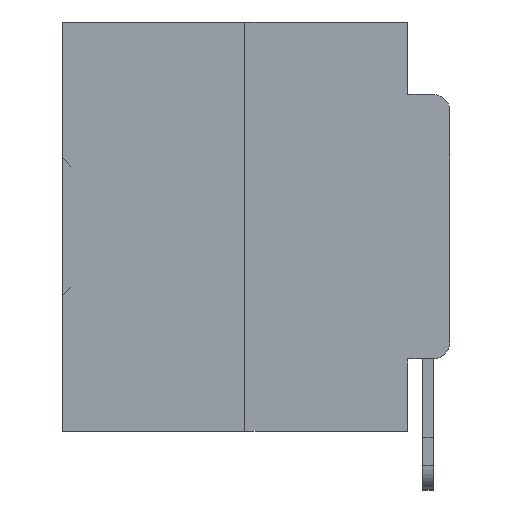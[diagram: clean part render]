
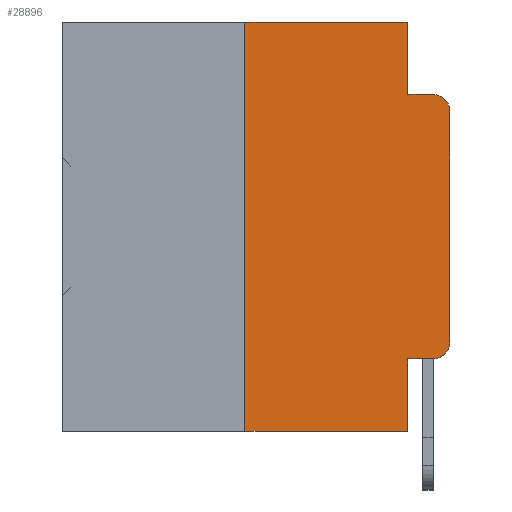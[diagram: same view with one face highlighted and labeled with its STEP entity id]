
A CAD part, left-side view. The second image highlights one B-rep face of the part: STEP entity #28896.
In plain terms, the highlighted planar face has unit normal (-1, 0, 0).
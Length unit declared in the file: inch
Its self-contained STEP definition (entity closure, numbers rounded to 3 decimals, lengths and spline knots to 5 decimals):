
#192 = DIRECTION ( 'NONE',  ( -1., 0., 0. ) ) ;
#407 = VERTEX_POINT ( 'NONE', #36374 ) ;
#588 = VERTEX_POINT ( 'NONE', #10167 ) ;
#618 = AXIS2_PLACEMENT_3D ( 'NONE', #33486, #6969, #27730 ) ;
#1060 = FACE_OUTER_BOUND ( 'NONE', #7384, .T. ) ;
#1232 = DIRECTION ( 'NONE',  ( 0., -1., 0. ) ) ;
#2127 = CARTESIAN_POINT ( 'NONE',  ( 0., 0.25, -0.5 ) ) ;
#2535 = CARTESIAN_POINT ( 'NONE',  ( 0., 0.02, -0.1085 ) ) ;
#4523 = CARTESIAN_POINT ( 'NONE',  ( 0., 0.02, -0.0885 ) ) ;
#4922 = CARTESIAN_POINT ( 'NONE',  ( 0., 0.051, 0. ) ) ;
#5551 = CARTESIAN_POINT ( 'NONE',  ( 0., 0.051, 0. ) ) ;
#5666 = DIRECTION ( 'NONE',  ( 0., 0., -1. ) ) ;
#5694 = AXIS2_PLACEMENT_3D ( 'NONE', #18422, #192, #21390 ) ;
#6969 = DIRECTION ( 'NONE',  ( 1., 0., 0. ) ) ;
#7015 = ORIENTED_EDGE ( 'NONE', *, *, #19990, .T. ) ;
#7384 = EDGE_LOOP ( 'NONE', ( #13612, #21499, #26997, #12244, #21073, #36648, #7015, #8926, #20641, #31150 ) ) ;
#8926 = ORIENTED_EDGE ( 'NONE', *, *, #18281, .F. ) ;
#9078 = DIRECTION ( 'NONE',  ( 0., -1., 0. ) ) ;
#9864 = VERTEX_POINT ( 'NONE', #4523 ) ;
#10167 = CARTESIAN_POINT ( 'NONE',  ( 0., 0.051, -0.5 ) ) ;
#10379 = CARTESIAN_POINT ( 'NONE',  ( 0., 0.051, -0.4115 ) ) ;
#10422 = CARTESIAN_POINT ( 'NONE',  ( 0., 0.051, 0. ) ) ;
#11445 = VERTEX_POINT ( 'NONE', #2127 ) ;
#12244 = ORIENTED_EDGE ( 'NONE', *, *, #34734, .F. ) ;
#12903 = VECTOR ( 'NONE', #1232, 39.37008 ) ;
#13021 = EDGE_CURVE ( 'NONE', #19128, #30905, #17056, .T. ) ;
#13612 = ORIENTED_EDGE ( 'NONE', *, *, #13021, .T. ) ;
#13676 = LINE ( 'NONE', #17434, #36222 ) ;
#15036 = EDGE_CURVE ( 'NONE', #30905, #9864, #26181, .T. ) ;
#16283 = EDGE_CURVE ( 'NONE', #11445, #407, #13676, .T. ) ;
#17056 = LINE ( 'NONE', #36546, #23977 ) ;
#17434 = CARTESIAN_POINT ( 'NONE',  ( 0., 0.25, 0. ) ) ;
#18281 = EDGE_CURVE ( 'NONE', #25551, #588, #29620, .T. ) ;
#18422 = CARTESIAN_POINT ( 'NONE',  ( 0., 0.02, -0.3915 ) ) ;
#18903 = PLANE ( 'NONE',  #618 ) ;
#19128 = VERTEX_POINT ( 'NONE', #24439 ) ;
#19990 = EDGE_CURVE ( 'NONE', #11445, #588, #25366, .T. ) ;
#20268 = EDGE_CURVE ( 'NONE', #25551, #32453, #20829, .T. ) ;
#20641 = ORIENTED_EDGE ( 'NONE', *, *, #20268, .T. ) ;
#20829 = LINE ( 'NONE', #10379, #12903 ) ;
#21073 = ORIENTED_EDGE ( 'NONE', *, *, #23882, .F. ) ;
#21390 = DIRECTION ( 'NONE',  ( 0., 0., -1. ) ) ;
#21456 = LINE ( 'NONE', #10422, #28306 ) ;
#21499 = ORIENTED_EDGE ( 'NONE', *, *, #15036, .T. ) ;
#21853 = CARTESIAN_POINT ( 'NONE',  ( 0., 0., -0.1085 ) ) ;
#22083 = VECTOR ( 'NONE', #22388, 39.37008 ) ;
#22388 = DIRECTION ( 'NONE',  ( 0., -1., 0. ) ) ;
#23063 = VERTEX_POINT ( 'NONE', #35932 ) ;
#23603 = DIRECTION ( 'NONE',  ( -1., 0., 0. ) ) ;
#23882 = EDGE_CURVE ( 'NONE', #407, #29100, #24645, .T. ) ;
#23977 = VECTOR ( 'NONE', #27792, 39.37008 ) ;
#24204 = EDGE_CURVE ( 'NONE', #32453, #19128, #29168, .T. ) ;
#24439 = CARTESIAN_POINT ( 'NONE',  ( 0., 0., -0.3915 ) ) ;
#24645 = LINE ( 'NONE', #36798, #31503 ) ;
#25366 = LINE ( 'NONE', #29759, #31302 ) ;
#25551 = VERTEX_POINT ( 'NONE', #32584 ) ;
#26181 = CIRCLE ( 'NONE', #32581, 0.02 ) ;
#26413 = DIRECTION ( 'NONE',  ( 0., 0., -1. ) ) ;
#26997 = ORIENTED_EDGE ( 'NONE', *, *, #32760, .F. ) ;
#27730 = DIRECTION ( 'NONE',  ( 0., 0., -1. ) ) ;
#27792 = DIRECTION ( 'NONE',  ( 0., 0., 1. ) ) ;
#28306 = VECTOR ( 'NONE', #34016, 39.37008 ) ;
#28896 = ADVANCED_FACE ( 'NONE', ( #1060 ), #18903, .F. ) ;
#29100 = VERTEX_POINT ( 'NONE', #4922 ) ;
#29168 = CIRCLE ( 'NONE', #5694, 0.02 ) ;
#29620 = LINE ( 'NONE', #5551, #36536 ) ;
#29759 = CARTESIAN_POINT ( 'NONE',  ( 0., 0.473, -0.5 ) ) ;
#30905 = VERTEX_POINT ( 'NONE', #21853 ) ;
#30991 = DIRECTION ( 'NONE',  ( 0., -1., 0. ) ) ;
#31058 = CARTESIAN_POINT ( 'NONE',  ( 0., 0.051, -0.0885 ) ) ;
#31150 = ORIENTED_EDGE ( 'NONE', *, *, #24204, .T. ) ;
#31302 = VECTOR ( 'NONE', #9078, 39.37008 ) ;
#31503 = VECTOR ( 'NONE', #30991, 39.37008 ) ;
#32453 = VERTEX_POINT ( 'NONE', #38404 ) ;
#32581 = AXIS2_PLACEMENT_3D ( 'NONE', #2535, #23603, #5666 ) ;
#32584 = CARTESIAN_POINT ( 'NONE',  ( 0., 0.051, -0.4115 ) ) ;
#32760 = EDGE_CURVE ( 'NONE', #23063, #9864, #37679, .T. ) ;
#33486 = CARTESIAN_POINT ( 'NONE',  ( 0., 0.473, 0. ) ) ;
#34016 = DIRECTION ( 'NONE',  ( 0., 0., -1. ) ) ;
#34734 = EDGE_CURVE ( 'NONE', #29100, #23063, #21456, .T. ) ;
#34999 = DIRECTION ( 'NONE',  ( 0., 0., 1. ) ) ;
#35932 = CARTESIAN_POINT ( 'NONE',  ( 0., 0.051, -0.0885 ) ) ;
#36222 = VECTOR ( 'NONE', #34999, 39.37008 ) ;
#36374 = CARTESIAN_POINT ( 'NONE',  ( 0., 0.25, 0. ) ) ;
#36536 = VECTOR ( 'NONE', #26413, 39.37008 ) ;
#36546 = CARTESIAN_POINT ( 'NONE',  ( 0., 0., 0. ) ) ;
#36648 = ORIENTED_EDGE ( 'NONE', *, *, #16283, .F. ) ;
#36798 = CARTESIAN_POINT ( 'NONE',  ( 0., 0.473, 0. ) ) ;
#37679 = LINE ( 'NONE', #31058, #22083 ) ;
#38404 = CARTESIAN_POINT ( 'NONE',  ( 0., 0.02, -0.4115 ) ) ;
